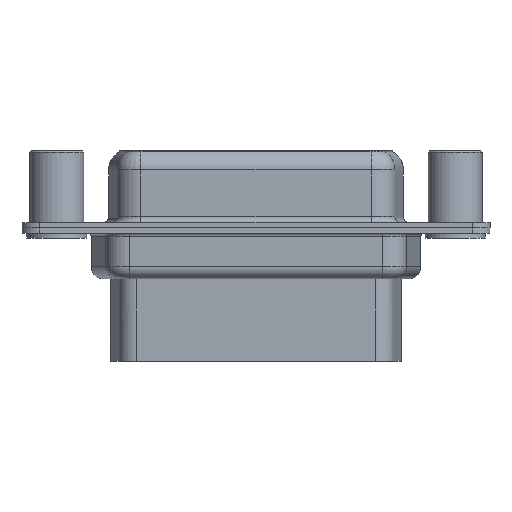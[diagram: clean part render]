
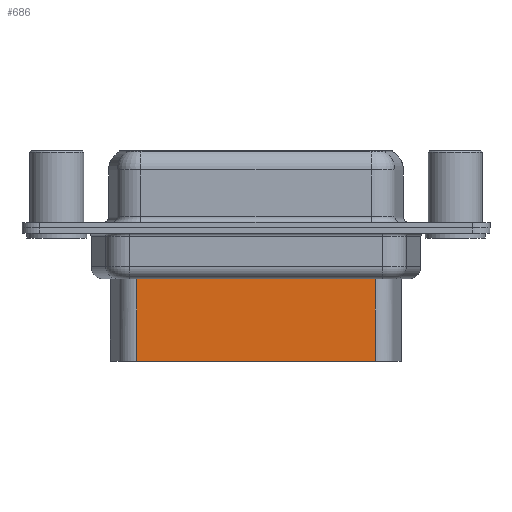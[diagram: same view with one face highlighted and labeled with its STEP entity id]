
A CAD part, front view. The second image highlights one B-rep face of the part: STEP entity #686.
In plain terms, the highlighted planar face has unit normal (0, -1, 0).
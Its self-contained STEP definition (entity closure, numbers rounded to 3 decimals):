
#303 = AXIS2_PLACEMENT_3D ( 'NONE', #320, #14851, #13731 ) ;
#320 = CARTESIAN_POINT ( 'NONE',  ( 6.681, -3.5, -3.1 ) ) ;
#686 = ADVANCED_FACE ( 'NONE', ( #12384 ), #13886, .T. ) ;
#733 = CARTESIAN_POINT ( 'NONE',  ( 6.434, -3.5, -4.097 ) ) ;
#750 = CARTESIAN_POINT ( 'NONE',  ( 6.681, -3.5, -11.15 ) ) ;
#879 = ORIENTED_EDGE ( 'NONE', *, *, #8507, .F. ) ;
#1269 = EDGE_CURVE ( 'NONE', #6468, #4360, #8212, .T. ) ;
#1401 = VECTOR ( 'NONE', #5682, 1000. ) ;
#1748 = VECTOR ( 'NONE', #7405, 1000. ) ;
#2099 = CARTESIAN_POINT ( 'NONE',  ( 6.681, -3.5, -11.15 ) ) ;
#2101 = EDGE_LOOP ( 'NONE', ( #879, #4868, #3888, #12593 ) ) ;
#2117 = EDGE_CURVE ( 'NONE', #2130, #7752, #6899, .T. ) ;
#2130 = VERTEX_POINT ( 'NONE', #15061 ) ;
#3888 = ORIENTED_EDGE ( 'NONE', *, *, #7330, .T. ) ;
#4360 = VERTEX_POINT ( 'NONE', #14310 ) ;
#4421 = VECTOR ( 'NONE', #9430, 1000. ) ;
#4469 = DIRECTION ( 'NONE',  ( -1., 0., 0. ) ) ;
#4868 = ORIENTED_EDGE ( 'NONE', *, *, #1269, .T. ) ;
#5682 = DIRECTION ( 'NONE',  ( -1., 0., 0. ) ) ;
#6309 = VECTOR ( 'NONE', #4469, 1000. ) ;
#6468 = VERTEX_POINT ( 'NONE', #15523 ) ;
#6899 = LINE ( 'NONE', #2099, #6309 ) ;
#7330 = EDGE_CURVE ( 'NONE', #4360, #7752, #15451, .T. ) ;
#7405 = DIRECTION ( 'NONE',  ( 0., 0., -1. ) ) ;
#7752 = VERTEX_POINT ( 'NONE', #750 ) ;
#8212 = LINE ( 'NONE', #733, #1401 ) ;
#8507 = EDGE_CURVE ( 'NONE', #6468, #2130, #11120, .T. ) ;
#9430 = DIRECTION ( 'NONE',  ( 0., 0., -1. ) ) ;
#9930 = CARTESIAN_POINT ( 'NONE',  ( 26.619, -3.5, -3.1 ) ) ;
#11120 = LINE ( 'NONE', #9930, #1748 ) ;
#12384 = FACE_OUTER_BOUND ( 'NONE', #2101, .T. ) ;
#12593 = ORIENTED_EDGE ( 'NONE', *, *, #2117, .F. ) ;
#13731 = DIRECTION ( 'NONE',  ( 1., 0., 0. ) ) ;
#13886 = PLANE ( 'NONE',  #303 ) ;
#14108 = CARTESIAN_POINT ( 'NONE',  ( 6.681, -3.5, -3.1 ) ) ;
#14310 = CARTESIAN_POINT ( 'NONE',  ( 6.681, -3.5, -4.097 ) ) ;
#14851 = DIRECTION ( 'NONE',  ( 0., -1., 0. ) ) ;
#15061 = CARTESIAN_POINT ( 'NONE',  ( 26.619, -3.5, -11.15 ) ) ;
#15451 = LINE ( 'NONE', #14108, #4421 ) ;
#15523 = CARTESIAN_POINT ( 'NONE',  ( 26.619, -3.5, -4.097 ) ) ;
